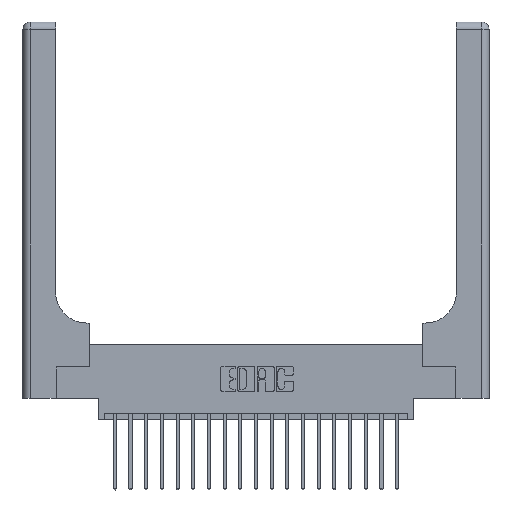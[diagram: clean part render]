
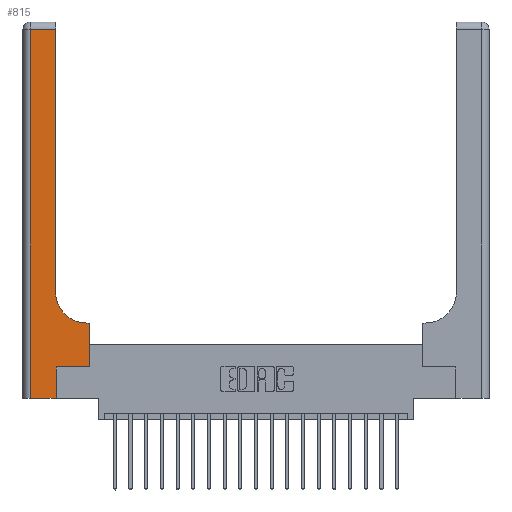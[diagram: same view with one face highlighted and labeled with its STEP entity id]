
A CAD part, top view. The second image highlights one B-rep face of the part: STEP entity #815.
In plain terms, the highlighted planar face has unit normal (0, 0, 1).
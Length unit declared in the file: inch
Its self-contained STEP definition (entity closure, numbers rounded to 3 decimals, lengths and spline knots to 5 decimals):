
#481 = EDGE_CURVE ( 'NONE', #10706, #15879, #12682, .T. ) ;
#607 = VERTEX_POINT ( 'NONE', #5850 ) ;
#815 = ADVANCED_FACE ( 'NONE', ( #16162 ), #7171, .F. ) ;
#1619 = DIRECTION ( 'NONE',  ( 0., 0., -1. ) ) ;
#2119 = CARTESIAN_POINT ( 'NONE',  ( 0.06, 2.94, 0.37 ) ) ;
#2805 = CARTESIAN_POINT ( 'NONE',  ( 0., 2.94, 0.37 ) ) ;
#2838 = VERTEX_POINT ( 'NONE', #13623 ) ;
#3140 = DIRECTION ( 'NONE',  ( -1., 0., 0. ) ) ;
#3186 = VECTOR ( 'NONE', #11655, 39.37008 ) ;
#3213 = AXIS2_PLACEMENT_3D ( 'NONE', #11310, #1619, #12908 ) ;
#3448 = CARTESIAN_POINT ( 'NONE',  ( 0.265, 0., 0.37 ) ) ;
#3754 = LINE ( 'NONE', #18016, #20354 ) ;
#3850 = ORIENTED_EDGE ( 'NONE', *, *, #7134, .T. ) ;
#4154 = DIRECTION ( 'NONE',  ( -1., 0., 0. ) ) ;
#4711 = LINE ( 'NONE', #2805, #12762 ) ;
#4713 = DIRECTION ( 'NONE',  ( 0., 0., -1. ) ) ;
#4887 = LINE ( 'NONE', #14471, #20461 ) ;
#5116 = ORIENTED_EDGE ( 'NONE', *, *, #16653, .T. ) ;
#5549 = CARTESIAN_POINT ( 'NONE',  ( 0., 3., 0.37 ) ) ;
#5850 = CARTESIAN_POINT ( 'NONE',  ( 0.26, 0.85, 0.37 ) ) ;
#5986 = CARTESIAN_POINT ( 'NONE',  ( 0.26, 2.94, 0.37 ) ) ;
#6108 = VERTEX_POINT ( 'NONE', #9579 ) ;
#6151 = ORIENTED_EDGE ( 'NONE', *, *, #18321, .T. ) ;
#6782 = DIRECTION ( 'NONE',  ( 0., 1., 0. ) ) ;
#6784 = CARTESIAN_POINT ( 'NONE',  ( 0.06, 3., 0.37 ) ) ;
#7134 = EDGE_CURVE ( 'NONE', #2838, #10303, #13605, .T. ) ;
#7171 = PLANE ( 'NONE',  #9601 ) ;
#7956 = EDGE_CURVE ( 'NONE', #15879, #2838, #16361, .T. ) ;
#8443 = CARTESIAN_POINT ( 'NONE',  ( 0.528, 0.6, 0.37 ) ) ;
#8925 = EDGE_LOOP ( 'NONE', ( #5116, #18431, #6151, #15179, #19943, #3850, #17201, #9707, #14429 ) ) ;
#9352 = DIRECTION ( 'NONE',  ( -1., 0., 0. ) ) ;
#9579 = CARTESIAN_POINT ( 'NONE',  ( 0.51, 0.6, 0.37 ) ) ;
#9600 = DIRECTION ( 'NONE',  ( 1., 0., 0. ) ) ;
#9601 = AXIS2_PLACEMENT_3D ( 'NONE', #5549, #4713, #4154 ) ;
#9707 = ORIENTED_EDGE ( 'NONE', *, *, #17616, .T. ) ;
#10303 = VERTEX_POINT ( 'NONE', #10582 ) ;
#10582 = CARTESIAN_POINT ( 'NONE',  ( 0.528, 0.25, 0.37 ) ) ;
#10706 = VERTEX_POINT ( 'NONE', #13133 ) ;
#10739 = VERTEX_POINT ( 'NONE', #8443 ) ;
#10975 = CARTESIAN_POINT ( 'NONE',  ( 0., 0., 0.37 ) ) ;
#11310 = CARTESIAN_POINT ( 'NONE',  ( 0.51, 0.85, 0.37 ) ) ;
#11441 = DIRECTION ( 'NONE',  ( 1., 0., 0. ) ) ;
#11495 = EDGE_CURVE ( 'NONE', #18908, #19290, #4711, .T. ) ;
#11655 = DIRECTION ( 'NONE',  ( 0., -1., 0. ) ) ;
#12117 = VECTOR ( 'NONE', #17933, 39.37008 ) ;
#12181 = CIRCLE ( 'NONE', #3213, 0.25 ) ;
#12682 = LINE ( 'NONE', #10975, #15425 ) ;
#12762 = VECTOR ( 'NONE', #9352, 39.37008 ) ;
#12800 = CARTESIAN_POINT ( 'NONE',  ( 0.26, 0.6, 0.37 ) ) ;
#12908 = DIRECTION ( 'NONE',  ( 1., 0., 0. ) ) ;
#13133 = CARTESIAN_POINT ( 'NONE',  ( 0.06, 0., 0.37 ) ) ;
#13201 = EDGE_CURVE ( 'NONE', #10303, #10739, #4887, .T. ) ;
#13605 = LINE ( 'NONE', #15248, #16870 ) ;
#13623 = CARTESIAN_POINT ( 'NONE',  ( 0.265, 0.25, 0.37 ) ) ;
#13941 = EDGE_CURVE ( 'NONE', #6108, #607, #12181, .T. ) ;
#14429 = ORIENTED_EDGE ( 'NONE', *, *, #13941, .T. ) ;
#14471 = CARTESIAN_POINT ( 'NONE',  ( 0.528, 0.25, 0.37 ) ) ;
#15179 = ORIENTED_EDGE ( 'NONE', *, *, #481, .T. ) ;
#15248 = CARTESIAN_POINT ( 'NONE',  ( 0.265, 0.25, 0.37 ) ) ;
#15304 = VECTOR ( 'NONE', #3140, 39.37008 ) ;
#15425 = VECTOR ( 'NONE', #11441, 39.37008 ) ;
#15879 = VERTEX_POINT ( 'NONE', #17699 ) ;
#16162 = FACE_OUTER_BOUND ( 'NONE', #8925, .T. ) ;
#16361 = LINE ( 'NONE', #3448, #12117 ) ;
#16653 = EDGE_CURVE ( 'NONE', #607, #18908, #3754, .T. ) ;
#16870 = VECTOR ( 'NONE', #9600, 39.37008 ) ;
#17201 = ORIENTED_EDGE ( 'NONE', *, *, #13201, .T. ) ;
#17616 = EDGE_CURVE ( 'NONE', #10739, #6108, #19077, .T. ) ;
#17699 = CARTESIAN_POINT ( 'NONE',  ( 0.265, 0., 0.37 ) ) ;
#17933 = DIRECTION ( 'NONE',  ( 0., 1., 0. ) ) ;
#18016 = CARTESIAN_POINT ( 'NONE',  ( 0.26, 3., 0.37 ) ) ;
#18321 = EDGE_CURVE ( 'NONE', #19290, #10706, #20303, .T. ) ;
#18431 = ORIENTED_EDGE ( 'NONE', *, *, #11495, .T. ) ;
#18908 = VERTEX_POINT ( 'NONE', #5986 ) ;
#19077 = LINE ( 'NONE', #12800, #15304 ) ;
#19290 = VERTEX_POINT ( 'NONE', #2119 ) ;
#19943 = ORIENTED_EDGE ( 'NONE', *, *, #7956, .T. ) ;
#20303 = LINE ( 'NONE', #6784, #3186 ) ;
#20354 = VECTOR ( 'NONE', #6782, 39.37008 ) ;
#20461 = VECTOR ( 'NONE', #20857, 39.37008 ) ;
#20857 = DIRECTION ( 'NONE',  ( 0., 1., 0. ) ) ;
